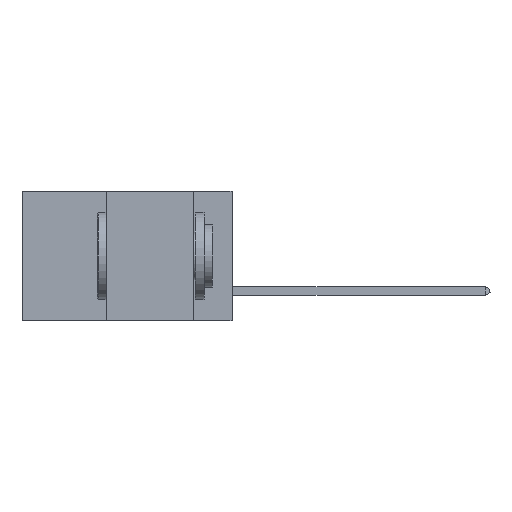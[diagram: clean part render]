
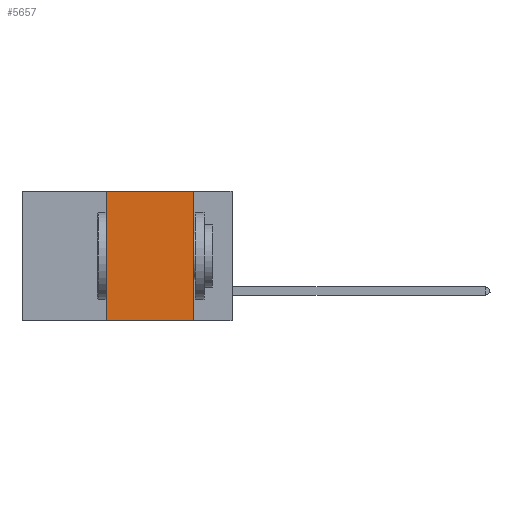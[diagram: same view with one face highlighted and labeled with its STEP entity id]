
A CAD part, left-side view. The second image highlights one B-rep face of the part: STEP entity #5657.
In plain terms, the highlighted planar face has unit normal (-1, 0, 0).
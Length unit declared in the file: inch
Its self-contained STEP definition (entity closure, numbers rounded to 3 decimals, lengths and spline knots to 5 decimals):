
#377 = EDGE_CURVE ( 'NONE', #2986, #4097, #9784, .T. ) ;
#1086 = VECTOR ( 'NONE', #10647, 39.37008 ) ;
#1532 = EDGE_CURVE ( 'NONE', #3843, #2986, #7262, .T. ) ;
#1660 = LINE ( 'NONE', #4233, #13210 ) ;
#1699 = CARTESIAN_POINT ( 'NONE',  ( 0., 0.11, -0.37 ) ) ;
#2195 = ORIENTED_EDGE ( 'NONE', *, *, #1532, .F. ) ;
#2986 = VERTEX_POINT ( 'NONE', #4616 ) ;
#3843 = VERTEX_POINT ( 'NONE', #8712 ) ;
#4097 = VERTEX_POINT ( 'NONE', #1699 ) ;
#4233 = CARTESIAN_POINT ( 'NONE',  ( 0., 0.36, 0. ) ) ;
#4316 = ORIENTED_EDGE ( 'NONE', *, *, #6918, .F. ) ;
#4616 = CARTESIAN_POINT ( 'NONE',  ( 0., 0.11, 0. ) ) ;
#4974 = CARTESIAN_POINT ( 'NONE',  ( 0., 0.6, -0.37 ) ) ;
#5027 = VERTEX_POINT ( 'NONE', #6579 ) ;
#5657 = ADVANCED_FACE ( 'NONE', ( #10945 ), #12659, .F. ) ;
#6036 = CARTESIAN_POINT ( 'NONE',  ( 0., 0.6, 0. ) ) ;
#6436 = VECTOR ( 'NONE', #8785, 39.37008 ) ;
#6579 = CARTESIAN_POINT ( 'NONE',  ( 0., 0.36, -0.37 ) ) ;
#6918 = EDGE_CURVE ( 'NONE', #5027, #3843, #1660, .T. ) ;
#7262 = LINE ( 'NONE', #9910, #12711 ) ;
#8347 = ORIENTED_EDGE ( 'NONE', *, *, #377, .F. ) ;
#8712 = CARTESIAN_POINT ( 'NONE',  ( 0., 0.36, 0. ) ) ;
#8752 = LINE ( 'NONE', #4974, #1086 ) ;
#8785 = DIRECTION ( 'NONE',  ( 0., 0., -1. ) ) ;
#9181 = DIRECTION ( 'NONE',  ( 0., 0., -1. ) ) ;
#9784 = LINE ( 'NONE', #13266, #6436 ) ;
#9910 = CARTESIAN_POINT ( 'NONE',  ( 0., 0.6, 0. ) ) ;
#10647 = DIRECTION ( 'NONE',  ( 0., -1., 0. ) ) ;
#10945 = FACE_OUTER_BOUND ( 'NONE', #12499, .T. ) ;
#11025 = DIRECTION ( 'NONE',  ( 0., -1., 0. ) ) ;
#11403 = ORIENTED_EDGE ( 'NONE', *, *, #11898, .T. ) ;
#11898 = EDGE_CURVE ( 'NONE', #5027, #4097, #8752, .T. ) ;
#12499 = EDGE_LOOP ( 'NONE', ( #8347, #2195, #4316, #11403 ) ) ;
#12659 = PLANE ( 'NONE',  #12666 ) ;
#12666 = AXIS2_PLACEMENT_3D ( 'NONE', #6036, #13879, #9181 ) ;
#12711 = VECTOR ( 'NONE', #11025, 39.37008 ) ;
#13210 = VECTOR ( 'NONE', #14328, 39.37008 ) ;
#13266 = CARTESIAN_POINT ( 'NONE',  ( 0., 0.11, 0. ) ) ;
#13879 = DIRECTION ( 'NONE',  ( 1., 0., 0. ) ) ;
#14328 = DIRECTION ( 'NONE',  ( 0., 0., 1. ) ) ;
